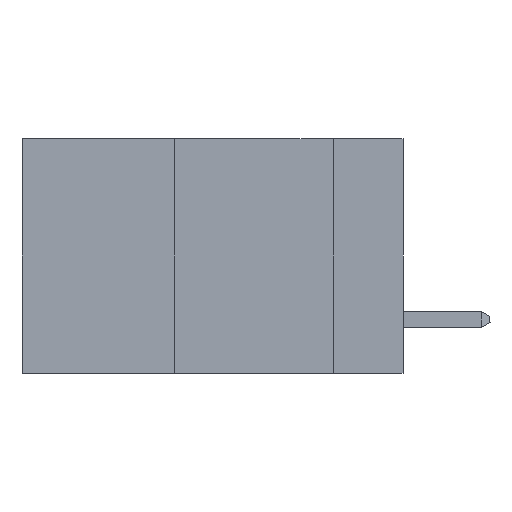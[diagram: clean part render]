
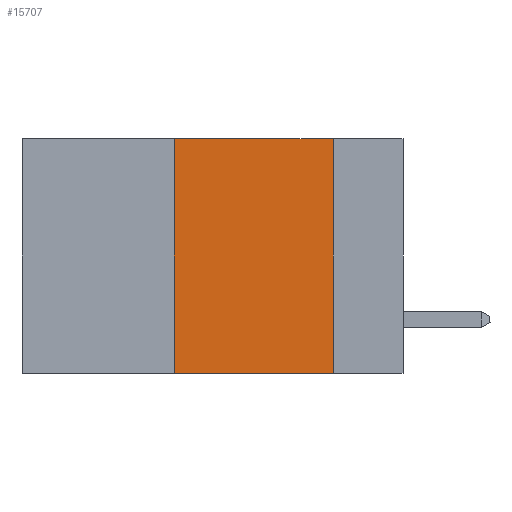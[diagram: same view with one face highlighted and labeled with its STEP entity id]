
A CAD part, left-side view. The second image highlights one B-rep face of the part: STEP entity #15707.
In plain terms, the highlighted planar face has unit normal (-1, 0, 0).
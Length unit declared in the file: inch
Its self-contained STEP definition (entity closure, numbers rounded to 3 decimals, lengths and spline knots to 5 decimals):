
#350 = VERTEX_POINT ( 'NONE', #24952 ) ;
#791 = VECTOR ( 'NONE', #12995, 39.37008 ) ;
#1887 = EDGE_CURVE ( 'NONE', #350, #3972, #39277, .T. ) ;
#3972 = VERTEX_POINT ( 'NONE', #12665 ) ;
#6428 = LINE ( 'NONE', #24492, #41603 ) ;
#7173 = CARTESIAN_POINT ( 'NONE',  ( 0., 0.36, -0.37 ) ) ;
#8220 = VERTEX_POINT ( 'NONE', #37108 ) ;
#8363 = VERTEX_POINT ( 'NONE', #7173 ) ;
#8982 = DIRECTION ( 'NONE',  ( 0., 0., 1. ) ) ;
#9194 = CARTESIAN_POINT ( 'NONE',  ( 0., 0.6, 0. ) ) ;
#12202 = DIRECTION ( 'NONE',  ( 1., 0., 0. ) ) ;
#12665 = CARTESIAN_POINT ( 'NONE',  ( 0., 0.11, 0. ) ) ;
#12995 = DIRECTION ( 'NONE',  ( 0., 0., -1. ) ) ;
#13212 = ORIENTED_EDGE ( 'NONE', *, *, #41662, .F. ) ;
#15062 = CARTESIAN_POINT ( 'NONE',  ( 0., 0.36, 0. ) ) ;
#15537 = DIRECTION ( 'NONE',  ( 0., 0., -1. ) ) ;
#15707 = ADVANCED_FACE ( 'NONE', ( #16303 ), #38483, .F. ) ;
#16303 = FACE_OUTER_BOUND ( 'NONE', #27628, .T. ) ;
#19863 = LINE ( 'NONE', #15062, #31229 ) ;
#24492 = CARTESIAN_POINT ( 'NONE',  ( 0., 0.6, -0.37 ) ) ;
#24952 = CARTESIAN_POINT ( 'NONE',  ( 0., 0.36, 0. ) ) ;
#26047 = ORIENTED_EDGE ( 'NONE', *, *, #35500, .T. ) ;
#26120 = CARTESIAN_POINT ( 'NONE',  ( 0., 0.11, 0. ) ) ;
#27628 = EDGE_LOOP ( 'NONE', ( #37037, #31845, #13212, #26047 ) ) ;
#28192 = LINE ( 'NONE', #26120, #791 ) ;
#31229 = VECTOR ( 'NONE', #8982, 39.37008 ) ;
#31845 = ORIENTED_EDGE ( 'NONE', *, *, #1887, .F. ) ;
#34115 = EDGE_CURVE ( 'NONE', #3972, #8220, #28192, .T. ) ;
#34464 = DIRECTION ( 'NONE',  ( 0., -1., 0. ) ) ;
#35500 = EDGE_CURVE ( 'NONE', #8363, #8220, #6428, .T. ) ;
#37037 = ORIENTED_EDGE ( 'NONE', *, *, #34115, .F. ) ;
#37108 = CARTESIAN_POINT ( 'NONE',  ( 0., 0.11, -0.37 ) ) ;
#37191 = VECTOR ( 'NONE', #41507, 39.37008 ) ;
#38483 = PLANE ( 'NONE',  #40101 ) ;
#39277 = LINE ( 'NONE', #40904, #37191 ) ;
#40101 = AXIS2_PLACEMENT_3D ( 'NONE', #9194, #12202, #15537 ) ;
#40904 = CARTESIAN_POINT ( 'NONE',  ( 0., 0.6, 0. ) ) ;
#41507 = DIRECTION ( 'NONE',  ( 0., -1., 0. ) ) ;
#41603 = VECTOR ( 'NONE', #34464, 39.37008 ) ;
#41662 = EDGE_CURVE ( 'NONE', #8363, #350, #19863, .T. ) ;
